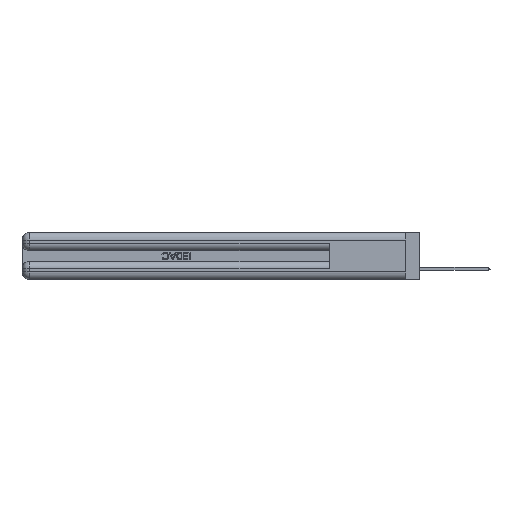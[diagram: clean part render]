
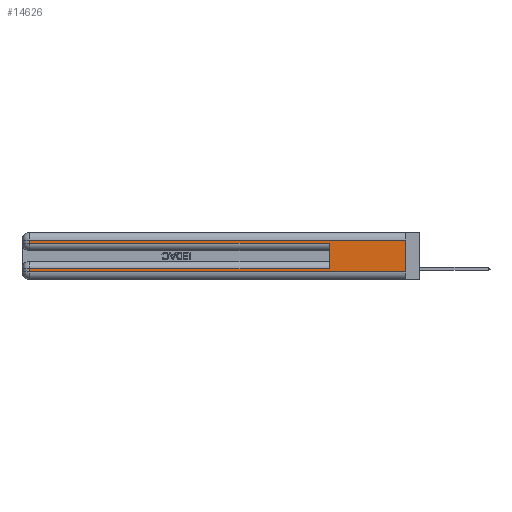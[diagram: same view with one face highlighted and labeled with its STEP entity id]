
A CAD part, left-side view. The second image highlights one B-rep face of the part: STEP entity #14626.
In plain terms, the highlighted planar face has unit normal (-1, 0, 0).
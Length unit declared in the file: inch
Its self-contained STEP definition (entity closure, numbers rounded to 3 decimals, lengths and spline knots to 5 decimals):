
#936 = CARTESIAN_POINT ( 'NONE',  ( 0., 2.94, 0.31 ) ) ;
#1987 = LINE ( 'NONE', #20523, #9100 ) ;
#3900 = ORIENTED_EDGE ( 'NONE', *, *, #37226, .F. ) ;
#4212 = ORIENTED_EDGE ( 'NONE', *, *, #24619, .F. ) ;
#4598 = VERTEX_POINT ( 'NONE', #936 ) ;
#4972 = EDGE_CURVE ( 'NONE', #38177, #29525, #17608, .T. ) ;
#5095 = CARTESIAN_POINT ( 'NONE',  ( 0., 0., 0.06 ) ) ;
#7598 = LINE ( 'NONE', #13846, #31805 ) ;
#7869 = DIRECTION ( 'NONE',  ( 0., 0., -1. ) ) ;
#8264 = VECTOR ( 'NONE', #16706, 39.37008 ) ;
#8880 = DIRECTION ( 'NONE',  ( 0., 0., -1. ) ) ;
#9100 = VECTOR ( 'NONE', #27598, 39.37008 ) ;
#12573 = VECTOR ( 'NONE', #32783, 39.37008 ) ;
#13205 = LINE ( 'NONE', #24171, #39609 ) ;
#13318 = CARTESIAN_POINT ( 'NONE',  ( 0., 0., 0.285 ) ) ;
#13650 = CARTESIAN_POINT ( 'NONE',  ( 0., 2.94, 0.285 ) ) ;
#13846 = CARTESIAN_POINT ( 'NONE',  ( 0., 2.94, 0.37 ) ) ;
#14260 = ORIENTED_EDGE ( 'NONE', *, *, #41308, .T. ) ;
#14626 = ADVANCED_FACE ( 'NONE', ( #15210 ), #41908, .F. ) ;
#14954 = DIRECTION ( 'NONE',  ( 0., -1., 0. ) ) ;
#15210 = FACE_OUTER_BOUND ( 'NONE', #17367, .T. ) ;
#15835 = VERTEX_POINT ( 'NONE', #44846 ) ;
#16706 = DIRECTION ( 'NONE',  ( 0., -1., 0. ) ) ;
#17099 = EDGE_CURVE ( 'NONE', #4598, #38177, #7598, .T. ) ;
#17367 = EDGE_LOOP ( 'NONE', ( #4212, #31584, #33510, #20326, #3900, #31971, #14260, #42311 ) ) ;
#17608 = LINE ( 'NONE', #13318, #8264 ) ;
#17919 = AXIS2_PLACEMENT_3D ( 'NONE', #35263, #24336, #38482 ) ;
#18592 = CARTESIAN_POINT ( 'NONE',  ( 0., 0.6, 0.285 ) ) ;
#19277 = LINE ( 'NONE', #23013, #31410 ) ;
#20326 = ORIENTED_EDGE ( 'NONE', *, *, #4972, .T. ) ;
#20523 = CARTESIAN_POINT ( 'NONE',  ( 0., 0., 0.085 ) ) ;
#21264 = CARTESIAN_POINT ( 'NONE',  ( 0., 0., 0.31 ) ) ;
#22695 = VERTEX_POINT ( 'NONE', #29762 ) ;
#23013 = CARTESIAN_POINT ( 'NONE',  ( 0., 0., 0.37 ) ) ;
#23620 = VECTOR ( 'NONE', #14954, 39.37008 ) ;
#24171 = CARTESIAN_POINT ( 'NONE',  ( 0., 0., 0.31 ) ) ;
#24336 = DIRECTION ( 'NONE',  ( 1., 0., 0. ) ) ;
#24619 = EDGE_CURVE ( 'NONE', #42419, #15835, #19277, .T. ) ;
#25276 = VERTEX_POINT ( 'NONE', #37955 ) ;
#25402 = VECTOR ( 'NONE', #7869, 39.37008 ) ;
#25519 = CARTESIAN_POINT ( 'NONE',  ( 0., 2.94, 0.37 ) ) ;
#27158 = EDGE_CURVE ( 'NONE', #32418, #22695, #1987, .T. ) ;
#27598 = DIRECTION ( 'NONE',  ( 0., 1., 0. ) ) ;
#29525 = VERTEX_POINT ( 'NONE', #18592 ) ;
#29762 = CARTESIAN_POINT ( 'NONE',  ( 0., 2.94, 0.085 ) ) ;
#31393 = DIRECTION ( 'NONE',  ( 0., 1., 0. ) ) ;
#31410 = VECTOR ( 'NONE', #8880, 39.37008 ) ;
#31584 = ORIENTED_EDGE ( 'NONE', *, *, #42482, .T. ) ;
#31680 = DIRECTION ( 'NONE',  ( 0., 0., -1. ) ) ;
#31695 = EDGE_CURVE ( 'NONE', #25276, #15835, #44563, .T. ) ;
#31805 = VECTOR ( 'NONE', #31680, 39.37008 ) ;
#31971 = ORIENTED_EDGE ( 'NONE', *, *, #27158, .T. ) ;
#32418 = VERTEX_POINT ( 'NONE', #45333 ) ;
#32783 = DIRECTION ( 'NONE',  ( 0., 0., 1. ) ) ;
#33510 = ORIENTED_EDGE ( 'NONE', *, *, #17099, .T. ) ;
#35263 = CARTESIAN_POINT ( 'NONE',  ( 0., 0., 0.37 ) ) ;
#35681 = LINE ( 'NONE', #39281, #12573 ) ;
#37226 = EDGE_CURVE ( 'NONE', #32418, #29525, #35681, .T. ) ;
#37955 = CARTESIAN_POINT ( 'NONE',  ( 0., 2.94, 0.06 ) ) ;
#38177 = VERTEX_POINT ( 'NONE', #13650 ) ;
#38482 = DIRECTION ( 'NONE',  ( 0., 0., -1. ) ) ;
#39281 = CARTESIAN_POINT ( 'NONE',  ( 0., 0.6, 0.145 ) ) ;
#39609 = VECTOR ( 'NONE', #31393, 39.37008 ) ;
#41308 = EDGE_CURVE ( 'NONE', #22695, #25276, #41951, .T. ) ;
#41908 = PLANE ( 'NONE',  #17919 ) ;
#41951 = LINE ( 'NONE', #25519, #25402 ) ;
#42311 = ORIENTED_EDGE ( 'NONE', *, *, #31695, .T. ) ;
#42419 = VERTEX_POINT ( 'NONE', #21264 ) ;
#42482 = EDGE_CURVE ( 'NONE', #42419, #4598, #13205, .T. ) ;
#44563 = LINE ( 'NONE', #5095, #23620 ) ;
#44846 = CARTESIAN_POINT ( 'NONE',  ( 0., 0., 0.06 ) ) ;
#45333 = CARTESIAN_POINT ( 'NONE',  ( 0., 0.6, 0.085 ) ) ;
